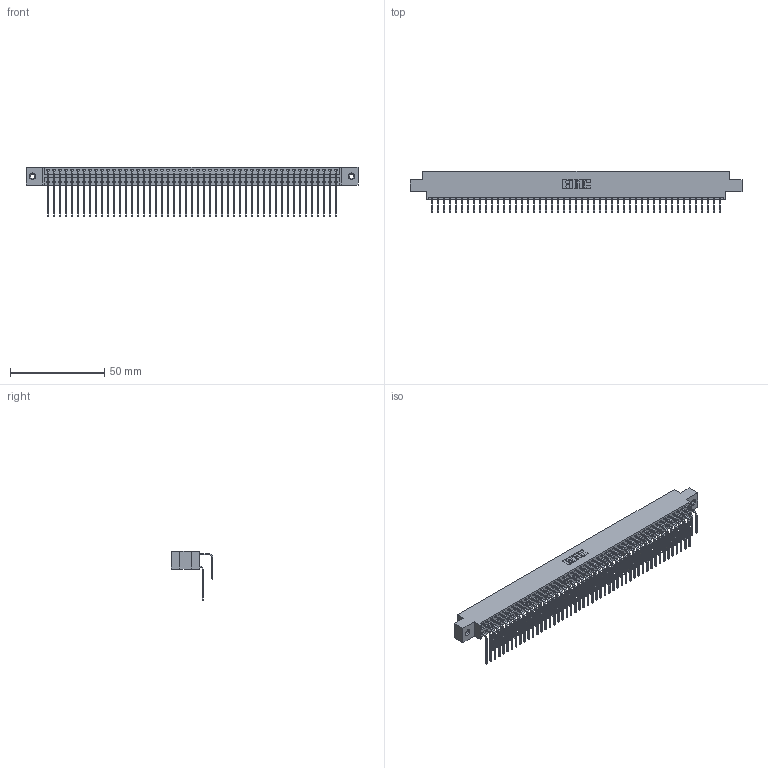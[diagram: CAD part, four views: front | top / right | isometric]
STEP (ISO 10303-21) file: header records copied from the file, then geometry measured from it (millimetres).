
FILE_DESCRIPTION (( 'STEP AP203' ), '1' );
FILE_NAME ('346-098-558-808.STEP', '2018-08-30T09:37:12', ( '' ), ( '' ), 'SwSTEP 2.0', 'SolidWorks 2016', '' );
FILE_SCHEMA (( 'CONFIG_CONTROL_DESIGN' ));
Length unit declared in the file: inch
Products named in the file (5): 346-098-558-808; 346 Part_0.170 Offset - 0.156 Dia-TI; 345-292-001_558 559 Tail - 1; 345-292-001_558 Tail - 2; 345-250-001_345-250-003-102
Assembly tree (101 placements, depth 2):
  346-098-558-808
    346 Part_0.170 Offset - 0.156 Dia-TI
    345-292-001_558 559 Tail - 1  x49
    345-292-001_558 Tail - 2  x49
    345-250-001_345-250-003-102  x2
Bounding box: 176.15 x 22.16 x 26.16 mm (x, y, z)
Volume: 1546.6 mm3
Topology: 100 solids, 102 shells, 5478 faces, 16255 edges, 10698 vertices
Faces by surface type: plane 3738, cylinder 1724, cone 12, torus 4
Entity records: 34138 total; most frequent: CARTESIAN_POINT 5654, ORIENTED_EDGE 5530, DIRECTION 5031, EDGE_CURVE 2765, VECTOR 2377, LINE 2377, VERTEX_POINT 1836, AXIS2_PLACEMENT_3D 1327
